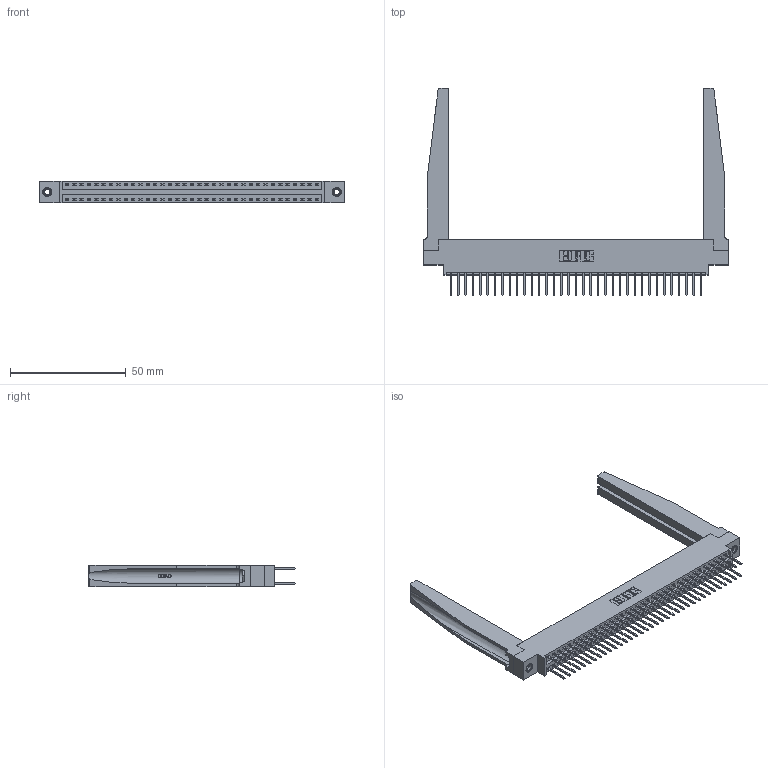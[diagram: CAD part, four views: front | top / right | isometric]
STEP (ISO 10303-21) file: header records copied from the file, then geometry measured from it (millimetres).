
FILE_DESCRIPTION (( 'STEP AP203' ), '1' );
FILE_NAME ('346-070-526-878.STEP', '2022-05-24T21:27:15', ( '' ), ( '' ), 'SwSTEP 2.0', 'SolidWorks 2020', '' );
FILE_SCHEMA (( 'CONFIG_CONTROL_DESIGN' ));
Length unit declared in the file: inch
Products named in the file (5): 346-220-078_345-220-078; 346-070-526-878; 345-250-001_345-250-001-102; 346 Part_0.170 Offset - 0.156 Dia-TH; 345-292-001_345-293-126
Assembly tree (75 placements, depth 2):
  346-070-526-878
    346 Part_0.170 Offset - 0.156 Dia-TH
    345-292-001_345-293-126  x70
    346-220-078_345-220-078  x2
    345-250-001_345-250-001-102  x2
Bounding box: 131.7 x 89.41 x 9.4 mm (x, y, z)
Volume: 19638.9 mm3; surface area: 24653.7 mm2
Topology: 75 solids, 75 shells, 4014 faces, 11835 edges, 7786 vertices
Faces by surface type: plane 2686, cylinder 1276, bspline 36, cone 12, torus 4
Entity records: 29098 total; most frequent: CARTESIAN_POINT 5749, ORIENTED_EDGE 4570, DIRECTION 4103, EDGE_CURVE 2285, LINE 1919, VECTOR 1919, VERTEX_POINT 1516, AXIS2_PLACEMENT_3D 1092
